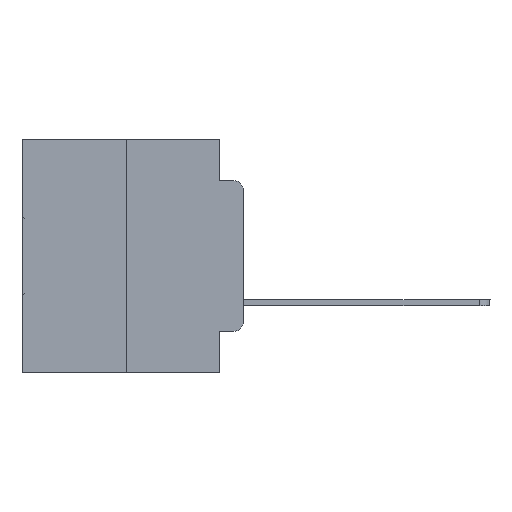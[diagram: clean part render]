
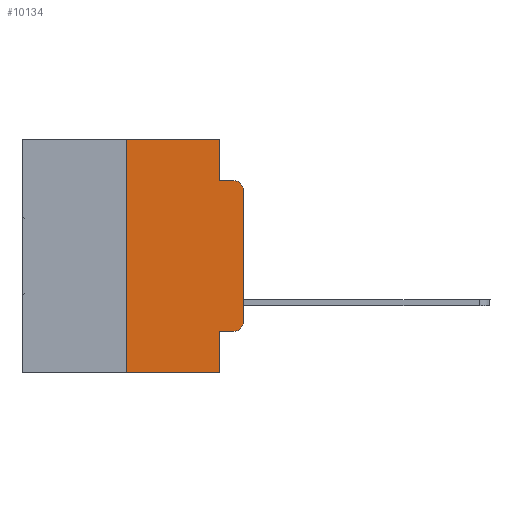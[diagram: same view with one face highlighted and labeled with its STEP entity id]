
A CAD part, left-side view. The second image highlights one B-rep face of the part: STEP entity #10134.
In plain terms, the highlighted planar face has unit normal (-1, 0, 0).
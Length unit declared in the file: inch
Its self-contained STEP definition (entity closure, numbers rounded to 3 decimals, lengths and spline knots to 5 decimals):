
#687 = DIRECTION ( 'NONE',  ( 1., 0., 0. ) ) ;
#1311 = ORIENTED_EDGE ( 'NONE', *, *, #26679, .T. ) ;
#1324 = CARTESIAN_POINT ( 'NONE',  ( 0., 0.25, -0.5 ) ) ;
#1811 = DIRECTION ( 'NONE',  ( 0., -1., 0. ) ) ;
#2371 = VERTEX_POINT ( 'NONE', #15763 ) ;
#2801 = CARTESIAN_POINT ( 'NONE',  ( 0., 0.02, -0.0885 ) ) ;
#3398 = VERTEX_POINT ( 'NONE', #2801 ) ;
#3804 = AXIS2_PLACEMENT_3D ( 'NONE', #18167, #8280, #5843 ) ;
#3862 = ORIENTED_EDGE ( 'NONE', *, *, #9018, .F. ) ;
#4063 = VECTOR ( 'NONE', #18203, 39.37008 ) ;
#4185 = CARTESIAN_POINT ( 'NONE',  ( 0., 0., 0. ) ) ;
#4737 = VERTEX_POINT ( 'NONE', #11055 ) ;
#4939 = ORIENTED_EDGE ( 'NONE', *, *, #9775, .F. ) ;
#5843 = DIRECTION ( 'NONE',  ( 0., 0., -1. ) ) ;
#6318 = EDGE_CURVE ( 'NONE', #12622, #2371, #16402, .T. ) ;
#8153 = EDGE_CURVE ( 'NONE', #27706, #10578, #30606, .T. ) ;
#8280 = DIRECTION ( 'NONE',  ( -1., 0., 0. ) ) ;
#8496 = ORIENTED_EDGE ( 'NONE', *, *, #16788, .F. ) ;
#9018 = EDGE_CURVE ( 'NONE', #4737, #19172, #26386, .T. ) ;
#9241 = CARTESIAN_POINT ( 'NONE',  ( 0., 0.051, 0. ) ) ;
#9291 = AXIS2_PLACEMENT_3D ( 'NONE', #25068, #687, #20070 ) ;
#9735 = EDGE_CURVE ( 'NONE', #26232, #12622, #29687, .T. ) ;
#9775 = EDGE_CURVE ( 'NONE', #15360, #4737, #10484, .T. ) ;
#10134 = ADVANCED_FACE ( 'NONE', ( #16889 ), #27181, .F. ) ;
#10484 = LINE ( 'NONE', #25258, #4063 ) ;
#10578 = VERTEX_POINT ( 'NONE', #21510 ) ;
#10602 = VECTOR ( 'NONE', #22039, 39.37008 ) ;
#11055 = CARTESIAN_POINT ( 'NONE',  ( 0., 0.25, 0. ) ) ;
#11223 = CARTESIAN_POINT ( 'NONE',  ( 0., 0.051, -0.0885 ) ) ;
#11634 = CARTESIAN_POINT ( 'NONE',  ( 0., 0.473, 0. ) ) ;
#11661 = LINE ( 'NONE', #9241, #17296 ) ;
#12555 = CARTESIAN_POINT ( 'NONE',  ( 0., 0., -0.3915 ) ) ;
#12622 = VERTEX_POINT ( 'NONE', #12555 ) ;
#12854 = ORIENTED_EDGE ( 'NONE', *, *, #6318, .T. ) ;
#13043 = DIRECTION ( 'NONE',  ( 0., -1., 0. ) ) ;
#13162 = LINE ( 'NONE', #29449, #23727 ) ;
#13779 = DIRECTION ( 'NONE',  ( 0., -1., 0. ) ) ;
#13865 = CARTESIAN_POINT ( 'NONE',  ( 0., 0.02, -0.4115 ) ) ;
#14184 = ORIENTED_EDGE ( 'NONE', *, *, #22350, .T. ) ;
#14321 = CIRCLE ( 'NONE', #3804, 0.02 ) ;
#14433 = VERTEX_POINT ( 'NONE', #11223 ) ;
#14725 = VECTOR ( 'NONE', #1811, 39.37008 ) ;
#14858 = LINE ( 'NONE', #29806, #15615 ) ;
#15360 = VERTEX_POINT ( 'NONE', #1324 ) ;
#15615 = VECTOR ( 'NONE', #22752, 39.37008 ) ;
#15763 = CARTESIAN_POINT ( 'NONE',  ( 0., 0., -0.1085 ) ) ;
#16391 = ORIENTED_EDGE ( 'NONE', *, *, #9735, .T. ) ;
#16402 = LINE ( 'NONE', #4185, #28051 ) ;
#16788 = EDGE_CURVE ( 'NONE', #19172, #14433, #11661, .T. ) ;
#16889 = FACE_OUTER_BOUND ( 'NONE', #21117, .T. ) ;
#17296 = VECTOR ( 'NONE', #23888, 39.37008 ) ;
#18052 = ORIENTED_EDGE ( 'NONE', *, *, #8153, .F. ) ;
#18167 = CARTESIAN_POINT ( 'NONE',  ( 0., 0.02, -0.1085 ) ) ;
#18203 = DIRECTION ( 'NONE',  ( 0., 0., 1. ) ) ;
#19041 = EDGE_CURVE ( 'NONE', #15360, #10578, #14858, .T. ) ;
#19172 = VERTEX_POINT ( 'NONE', #22178 ) ;
#19707 = AXIS2_PLACEMENT_3D ( 'NONE', #25430, #20661, #20766 ) ;
#20070 = DIRECTION ( 'NONE',  ( 0., 0., -1. ) ) ;
#20401 = ORIENTED_EDGE ( 'NONE', *, *, #29136, .F. ) ;
#20661 = DIRECTION ( 'NONE',  ( -1., 0., 0. ) ) ;
#20766 = DIRECTION ( 'NONE',  ( 0., 0., -1. ) ) ;
#21117 = EDGE_LOOP ( 'NONE', ( #12854, #14184, #20401, #8496, #3862, #4939, #31123, #18052, #1311, #16391 ) ) ;
#21350 = DIRECTION ( 'NONE',  ( 0., 0., 1. ) ) ;
#21510 = CARTESIAN_POINT ( 'NONE',  ( 0., 0.051, -0.5 ) ) ;
#21648 = CARTESIAN_POINT ( 'NONE',  ( 0., 0.051, 0. ) ) ;
#22039 = DIRECTION ( 'NONE',  ( 0., 0., -1. ) ) ;
#22178 = CARTESIAN_POINT ( 'NONE',  ( 0., 0.051, 0. ) ) ;
#22350 = EDGE_CURVE ( 'NONE', #2371, #3398, #14321, .T. ) ;
#22752 = DIRECTION ( 'NONE',  ( 0., -1., 0. ) ) ;
#22798 = VECTOR ( 'NONE', #13043, 39.37008 ) ;
#23727 = VECTOR ( 'NONE', #13779, 39.37008 ) ;
#23888 = DIRECTION ( 'NONE',  ( 0., 0., -1. ) ) ;
#24184 = CARTESIAN_POINT ( 'NONE',  ( 0., 0.051, -0.4115 ) ) ;
#25068 = CARTESIAN_POINT ( 'NONE',  ( 0., 0.473, 0. ) ) ;
#25258 = CARTESIAN_POINT ( 'NONE',  ( 0., 0.25, 0. ) ) ;
#25430 = CARTESIAN_POINT ( 'NONE',  ( 0., 0.02, -0.3915 ) ) ;
#26232 = VERTEX_POINT ( 'NONE', #13865 ) ;
#26386 = LINE ( 'NONE', #11634, #14725 ) ;
#26679 = EDGE_CURVE ( 'NONE', #27706, #26232, #13162, .T. ) ;
#27181 = PLANE ( 'NONE',  #9291 ) ;
#27353 = CARTESIAN_POINT ( 'NONE',  ( 0., 0.051, -0.0885 ) ) ;
#27706 = VERTEX_POINT ( 'NONE', #24184 ) ;
#28051 = VECTOR ( 'NONE', #21350, 39.37008 ) ;
#29136 = EDGE_CURVE ( 'NONE', #14433, #3398, #29180, .T. ) ;
#29180 = LINE ( 'NONE', #27353, #22798 ) ;
#29449 = CARTESIAN_POINT ( 'NONE',  ( 0., 0.051, -0.4115 ) ) ;
#29687 = CIRCLE ( 'NONE', #19707, 0.02 ) ;
#29806 = CARTESIAN_POINT ( 'NONE',  ( 0., 0.473, -0.5 ) ) ;
#30606 = LINE ( 'NONE', #21648, #10602 ) ;
#31123 = ORIENTED_EDGE ( 'NONE', *, *, #19041, .T. ) ;
